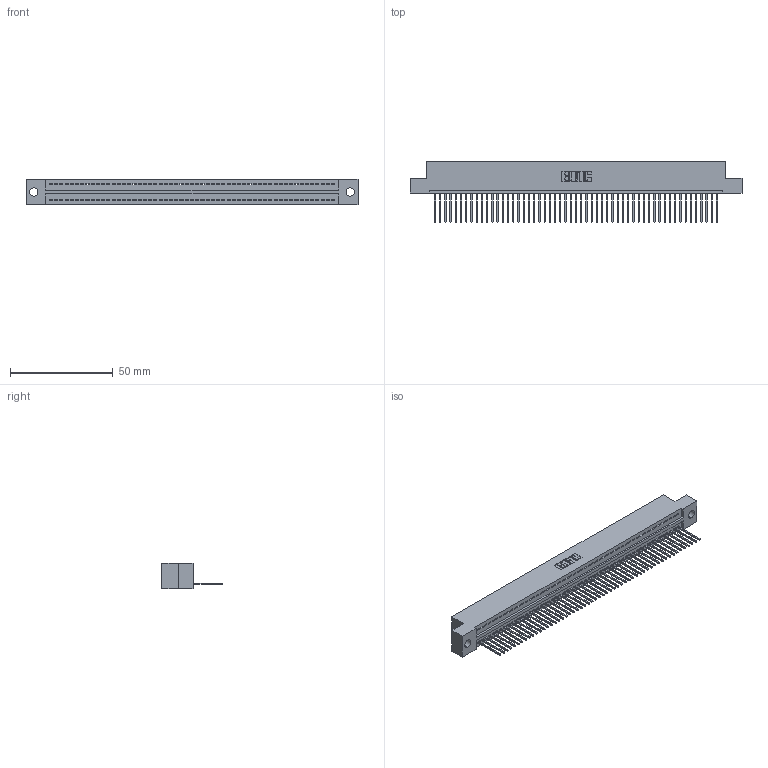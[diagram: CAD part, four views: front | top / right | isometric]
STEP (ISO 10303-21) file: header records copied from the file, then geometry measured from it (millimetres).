
FILE_DESCRIPTION (( 'STEP AP203' ), '1' );
FILE_NAME ('325-055-540-109.STEP', '2020-02-25T01:16:07', ( '' ), ( '' ), 'SwSTEP 2.0', 'SolidWorks 2016', '' );
FILE_SCHEMA (( 'CONFIG_CONTROL_DESIGN' ));
Length unit declared in the file: inch
Products named in the file (3): 325 Part_.160 TH; 325-055-540-109; 325-292-001_325-293-140
Assembly tree (56 placements, depth 2):
  325-055-540-109
    325 Part_.160 TH
    325-292-001_325-293-140  x55
Bounding box: 161.42 x 29.46 x 12.45 mm (x, y, z)
Volume: 20438.1 mm3; surface area: 22995.8 mm2
Topology: 56 solids, 56 shells, 3304 faces, 9991 edges, 6586 vertices
Faces by surface type: plane 2380, cylinder 924
Entity records: 31963 total; most frequent: CARTESIAN_POINT 5519, ORIENTED_EDGE 5510, DIRECTION 4629, EDGE_CURVE 2755, LINE 2627, VECTOR 2627, VERTEX_POINT 1834, AXIS2_PLACEMENT_3D 1001
